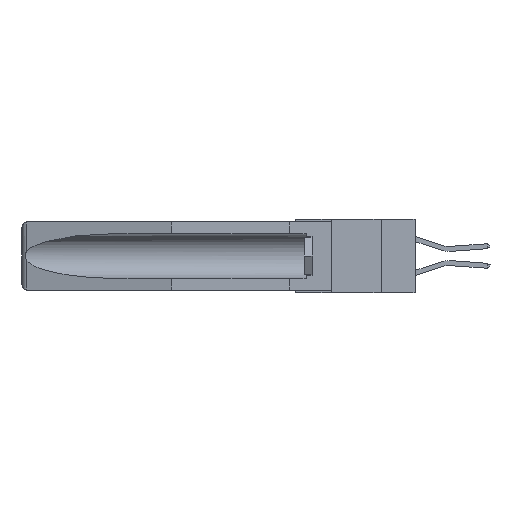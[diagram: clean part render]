
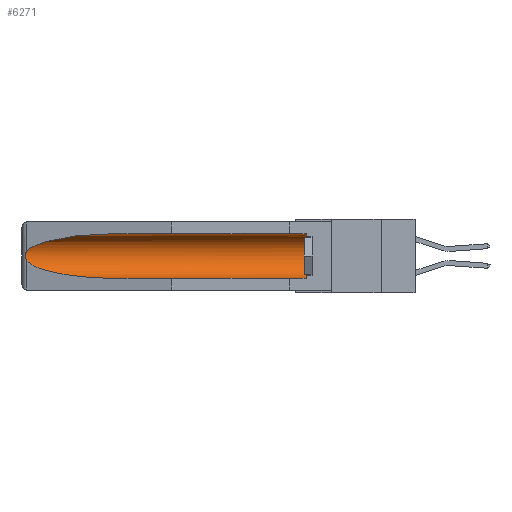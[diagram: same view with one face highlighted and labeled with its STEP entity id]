
A CAD part, left-side view. The second image highlights one B-rep face of the part: STEP entity #6271.
In plain terms, the highlighted cylindrical face has radius 2.857 mm (diameter 5.715 mm), a partial arc.
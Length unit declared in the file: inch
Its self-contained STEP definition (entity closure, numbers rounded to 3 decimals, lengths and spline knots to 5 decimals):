
#87 = CARTESIAN_POINT ( 'NONE',  ( 0.26537, 1.52718, -0.14972 ) ) ;
#608 = VERTEX_POINT ( 'NONE', #12153 ) ;
#1573 = CARTESIAN_POINT ( 'NONE',  ( 0.26597, 1.5296, -0.19026 ) ) ;
#1762 = FACE_OUTER_BOUND ( 'NONE', #14288, .T. ) ;
#1787 = CARTESIAN_POINT ( 'NONE',  ( 0.26537, 1.52718, -0.14972 ) ) ;
#1897 = VECTOR ( 'NONE', #14925, 39.37008 ) ;
#1987 = CARTESIAN_POINT ( 'NONE',  ( 0.21114, 1.30732, -0.284 ) ) ;
#2062 = CARTESIAN_POINT ( 'NONE',  ( 0.26537, 1.52718, -0.19328 ) ) ;
#2154 = EDGE_CURVE ( 'NONE', #5306, #14173, #18986, .T. ) ;
#2246 = ORIENTED_EDGE ( 'NONE', *, *, #2154, .F. ) ;
#2447 = LINE ( 'NONE', #4664, #13537 ) ;
#2841 = EDGE_CURVE ( 'NONE', #8287, #16884, #9536, .T. ) ;
#3101 = CARTESIAN_POINT ( 'NONE',  ( 0.155, -0.30754, -0.1715 ) ) ;
#3461 = CARTESIAN_POINT ( 'NONE',  ( 0.2675, 1.53308, -0.16763 ) ) ;
#3588 = CARTESIAN_POINT ( 'NONE',  ( 0.26537, 1.52718, -0.19328 ) ) ;
#3947 = ORIENTED_EDGE ( 'NONE', *, *, #17928, .T. ) ;
#3996 = ORIENTED_EDGE ( 'NONE', *, *, #2841, .T. ) ;
#4101 = CYLINDRICAL_SURFACE ( 'NONE', #9745, 0.1125 ) ;
#4136 = CARTESIAN_POINT ( 'NONE',  ( 0.155, -0.30754, -0.284 ) ) ;
#4518 = EDGE_CURVE ( 'NONE', #5306, #608, #17323, .T. ) ;
#4664 = CARTESIAN_POINT ( 'NONE',  ( 0.155, -0.30754, -0.059 ) ) ;
#4716 = CARTESIAN_POINT ( 'NONE',  ( 0.21114, 1.30732, -0.059 ) ) ;
#5111 = CARTESIAN_POINT ( 'NONE',  ( 0.26537, 1.52718, -0.14972 ) ) ;
#5306 = VERTEX_POINT ( 'NONE', #12122 ) ;
#5939 = DIRECTION ( 'NONE',  ( 0., 1., 0. ) ) ;
#6009 = EDGE_CURVE ( 'NONE', #13157, #8287, #18958, .T. ) ;
#6271 = ADVANCED_FACE ( 'NONE', ( #1762 ), #4101, .F. ) ;
#6324 = CARTESIAN_POINT ( 'NONE',  ( 0.155, 0.126, -0.1715 ) ) ;
#7343 = DIRECTION ( 'NONE',  ( 0., 0., 1. ) ) ;
#7660 = CARTESIAN_POINT ( 'NONE',  ( 0.25451, 1.48313, -0.09465 ) ) ;
#7805 = CARTESIAN_POINT ( 'NONE',  ( 0.155, 1.07973, -0.059 ) ) ;
#7940 = CARTESIAN_POINT ( 'NONE',  ( 0.25451, 1.48313, -0.24835 ) ) ;
#8097 =( BOUNDED_CURVE ( )  B_SPLINE_CURVE ( 3, ( #2062, #7940, #1987, #12214 ),
 .UNSPECIFIED., .F., .F. ) 
 B_SPLINE_CURVE_WITH_KNOTS ( ( 4, 4 ),
 ( 0.1948, 1.5708 ),
 .UNSPECIFIED. ) 
 CURVE ( )  GEOMETRIC_REPRESENTATION_ITEM ( )  RATIONAL_B_SPLINE_CURVE ( ( 1., 0.848, 0.848, 1. ) ) 
 REPRESENTATION_ITEM ( '' )  );
#8287 = VERTEX_POINT ( 'NONE', #5111 ) ;
#9012 = CARTESIAN_POINT ( 'NONE',  ( 0.155, 1.07973, -0.059 ) ) ;
#9127 = DIRECTION ( 'NONE',  ( 0., 1., 0. ) ) ;
#9187 = DIRECTION ( 'NONE',  ( 0., 0., 1. ) ) ;
#9536 = B_SPLINE_CURVE_WITH_KNOTS ( 'NONE', 3,
 ( #87, #14857, #12294, #13854, #3461, #10820, #10881, #13723, #1573, #3588 ),
 .UNSPECIFIED., .F., .F.,
 ( 4, 2, 2, 2, 4 ),
 ( 0., 0.00029, 0.00058, 0.00087, 0.00117 ),
 .UNSPECIFIED. ) ;
#9745 = AXIS2_PLACEMENT_3D ( 'NONE', #3101, #5939, #7343 ) ;
#9922 = CARTESIAN_POINT ( 'NONE',  ( 0.26537, 1.52718, -0.19328 ) ) ;
#10820 = CARTESIAN_POINT ( 'NONE',  ( 0.2675, 1.53308, -0.17534 ) ) ;
#10881 = CARTESIAN_POINT ( 'NONE',  ( 0.2673, 1.53269, -0.17917 ) ) ;
#12122 = CARTESIAN_POINT ( 'NONE',  ( 0.155, 0.126, -0.284 ) ) ;
#12153 = CARTESIAN_POINT ( 'NONE',  ( 0.155, 0.126, -0.059 ) ) ;
#12214 = CARTESIAN_POINT ( 'NONE',  ( 0.155, 1.07973, -0.284 ) ) ;
#12294 = CARTESIAN_POINT ( 'NONE',  ( 0.26654, 1.53092, -0.15636 ) ) ;
#12579 = ORIENTED_EDGE ( 'NONE', *, *, #18920, .T. ) ;
#13157 = VERTEX_POINT ( 'NONE', #9012 ) ;
#13537 = VECTOR ( 'NONE', #9127, 39.37008 ) ;
#13723 = CARTESIAN_POINT ( 'NONE',  ( 0.26655, 1.53094, -0.18657 ) ) ;
#13854 = CARTESIAN_POINT ( 'NONE',  ( 0.2673, 1.5327, -0.16383 ) ) ;
#14173 = VERTEX_POINT ( 'NONE', #14809 ) ;
#14270 = ORIENTED_EDGE ( 'NONE', *, *, #4518, .T. ) ;
#14288 = EDGE_LOOP ( 'NONE', ( #18120, #3996, #3947, #2246, #14270, #12579 ) ) ;
#14533 = AXIS2_PLACEMENT_3D ( 'NONE', #6324, #15159, #9187 ) ;
#14809 = CARTESIAN_POINT ( 'NONE',  ( 0.155, 1.07973, -0.284 ) ) ;
#14857 = CARTESIAN_POINT ( 'NONE',  ( 0.26597, 1.52961, -0.15275 ) ) ;
#14925 = DIRECTION ( 'NONE',  ( 0., 1., 0. ) ) ;
#15159 = DIRECTION ( 'NONE',  ( 0., -1., 0. ) ) ;
#16884 = VERTEX_POINT ( 'NONE', #9922 ) ;
#17323 = CIRCLE ( 'NONE', #14533, 0.1125 ) ;
#17928 = EDGE_CURVE ( 'NONE', #16884, #14173, #8097, .T. ) ;
#18120 = ORIENTED_EDGE ( 'NONE', *, *, #6009, .T. ) ;
#18920 = EDGE_CURVE ( 'NONE', #608, #13157, #2447, .T. ) ;
#18958 =( BOUNDED_CURVE ( )  B_SPLINE_CURVE ( 3, ( #7805, #4716, #7660, #1787 ),
 .UNSPECIFIED., .F., .F. ) 
 B_SPLINE_CURVE_WITH_KNOTS ( ( 4, 4 ),
 ( 4.71239, 6.08839 ),
 .UNSPECIFIED. ) 
 CURVE ( )  GEOMETRIC_REPRESENTATION_ITEM ( )  RATIONAL_B_SPLINE_CURVE ( ( 1., 0.848, 0.848, 1. ) ) 
 REPRESENTATION_ITEM ( '' )  );
#18986 = LINE ( 'NONE', #4136, #1897 ) ;
